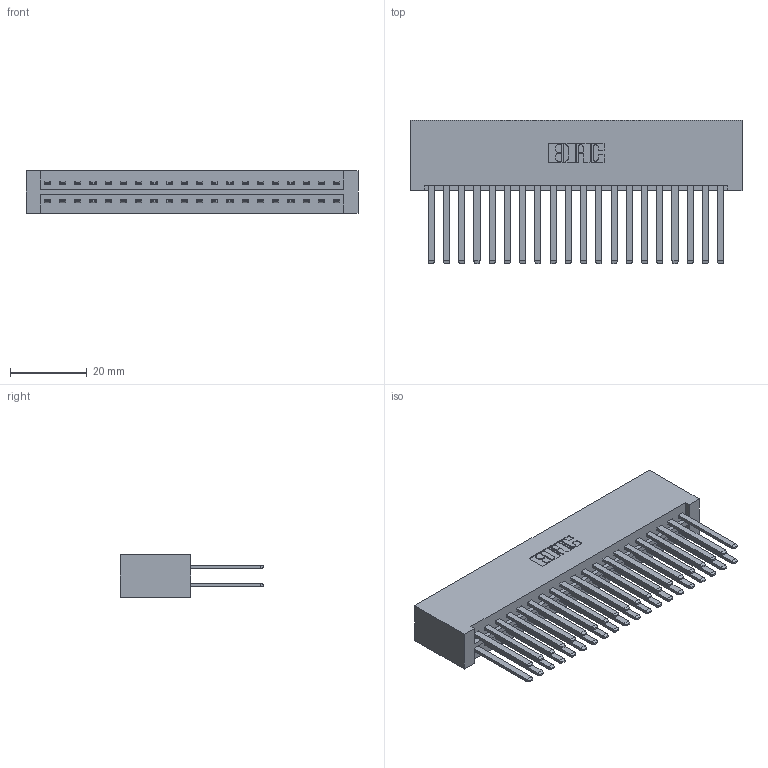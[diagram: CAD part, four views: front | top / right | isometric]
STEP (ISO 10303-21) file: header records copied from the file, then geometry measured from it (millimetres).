
FILE_DESCRIPTION (( 'STEP AP203' ), '1' );
FILE_NAME ('336-040-541-801.STEP', '2020-08-07T23:19:51', ( '' ), ( '' ), 'SwSTEP 2.0', 'SolidWorks 2020', '' );
FILE_SCHEMA (( 'CONFIG_CONTROL_DESIGN' ));
Length unit declared in the file: inch
Products named in the file (3): 336-290-001_336-290-541; 336-040-541-801; 336 Part_Lugless
Assembly tree (41 placements, depth 2):
  336-040-541-801
    336 Part_Lugless
    336-290-001_336-290-541  x40
Bounding box: 86.36 x 37.34 x 11.1 mm (x, y, z)
Volume: 14293.7 mm3; surface area: 18010.4 mm2
Topology: 41 solids, 41 shells, 1786 faces, 5367 edges, 3550 vertices
Faces by surface type: plane 1106, cylinder 680
Entity records: 17794 total; most frequent: CARTESIAN_POINT 3097, ORIENTED_EDGE 2934, DIRECTION 2571, EDGE_CURVE 1467, LINE 1343, VECTOR 1343, VERTEX_POINT 976, AXIS2_PLACEMENT_3D 614
